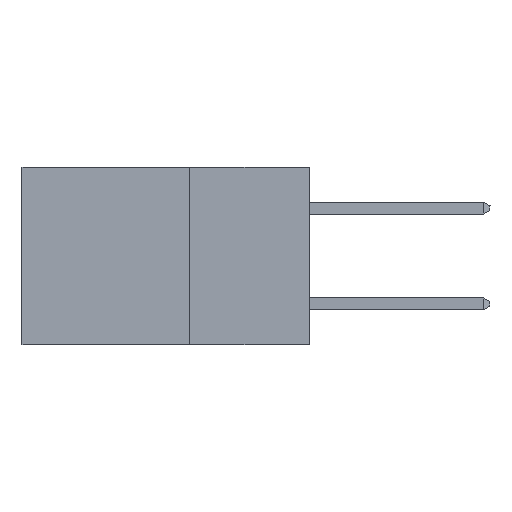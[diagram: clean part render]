
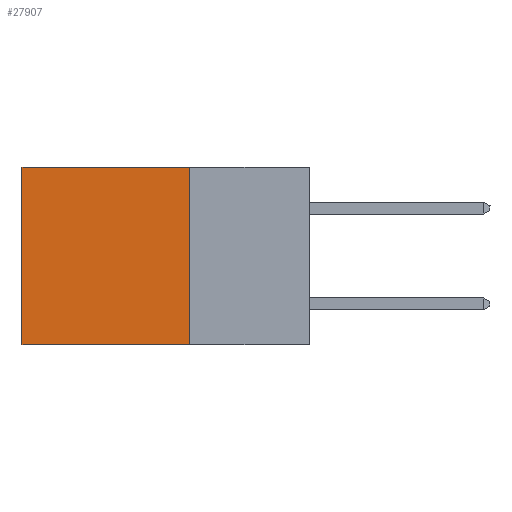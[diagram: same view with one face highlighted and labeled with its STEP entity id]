
A CAD part, left-side view. The second image highlights one B-rep face of the part: STEP entity #27907.
In plain terms, the highlighted planar face has unit normal (-1, 0, 0).
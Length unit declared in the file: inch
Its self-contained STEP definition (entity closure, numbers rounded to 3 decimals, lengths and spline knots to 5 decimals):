
#692 = DIRECTION ( 'NONE',  ( 0., 1., 0. ) ) ;
#735 = DIRECTION ( 'NONE',  ( 0., 0., -1. ) ) ;
#743 = LINE ( 'NONE', #29137, #6344 ) ;
#1001 = LINE ( 'NONE', #13153, #7374 ) ;
#2268 = LINE ( 'NONE', #11106, #8636 ) ;
#2664 = ORIENTED_EDGE ( 'NONE', *, *, #10425, .T. ) ;
#3133 = CARTESIAN_POINT ( 'NONE',  ( 0.2875, 0.25, -0.37 ) ) ;
#5380 = CARTESIAN_POINT ( 'NONE',  ( 0.2875, 0.25, 0. ) ) ;
#6344 = VECTOR ( 'NONE', #15412, 39.37008 ) ;
#7374 = VECTOR ( 'NONE', #17675, 39.37008 ) ;
#7667 = CARTESIAN_POINT ( 'NONE',  ( 0.2875, 0.25, 0. ) ) ;
#7876 = CARTESIAN_POINT ( 'NONE',  ( 0.2875, 0.25, 0. ) ) ;
#8636 = VECTOR ( 'NONE', #29568, 39.37008 ) ;
#9762 = AXIS2_PLACEMENT_3D ( 'NONE', #7876, #15025, #735 ) ;
#9885 = EDGE_CURVE ( 'NONE', #27851, #10485, #2268, .T. ) ;
#10425 = EDGE_CURVE ( 'NONE', #12982, #23091, #743, .T. ) ;
#10434 = EDGE_LOOP ( 'NONE', ( #2664, #13442, #20365, #20648 ) ) ;
#10485 = VERTEX_POINT ( 'NONE', #3133 ) ;
#11106 = CARTESIAN_POINT ( 'NONE',  ( 0.2875, 0.25, 0. ) ) ;
#12382 = FACE_OUTER_BOUND ( 'NONE', #10434, .T. ) ;
#12982 = VERTEX_POINT ( 'NONE', #28475 ) ;
#13153 = CARTESIAN_POINT ( 'NONE',  ( 0.2875, 0.25, -0.37 ) ) ;
#13442 = ORIENTED_EDGE ( 'NONE', *, *, #21476, .F. ) ;
#14136 = VECTOR ( 'NONE', #692, 39.37008 ) ;
#15025 = DIRECTION ( 'NONE',  ( 1., 0., 0. ) ) ;
#15412 = DIRECTION ( 'NONE',  ( 0., 0., -1. ) ) ;
#16298 = EDGE_CURVE ( 'NONE', #27851, #12982, #20197, .T. ) ;
#17675 = DIRECTION ( 'NONE',  ( 0., 1., 0. ) ) ;
#20197 = LINE ( 'NONE', #5380, #14136 ) ;
#20365 = ORIENTED_EDGE ( 'NONE', *, *, #9885, .F. ) ;
#20648 = ORIENTED_EDGE ( 'NONE', *, *, #16298, .T. ) ;
#21476 = EDGE_CURVE ( 'NONE', #10485, #23091, #1001, .T. ) ;
#23091 = VERTEX_POINT ( 'NONE', #28024 ) ;
#27851 = VERTEX_POINT ( 'NONE', #7667 ) ;
#27907 = ADVANCED_FACE ( 'NONE', ( #12382 ), #28715, .F. ) ;
#28024 = CARTESIAN_POINT ( 'NONE',  ( 0.2875, 0.6, -0.37 ) ) ;
#28475 = CARTESIAN_POINT ( 'NONE',  ( 0.2875, 0.6, 0. ) ) ;
#28715 = PLANE ( 'NONE',  #9762 ) ;
#29137 = CARTESIAN_POINT ( 'NONE',  ( 0.2875, 0.6, 0. ) ) ;
#29568 = DIRECTION ( 'NONE',  ( 0., 0., -1. ) ) ;
